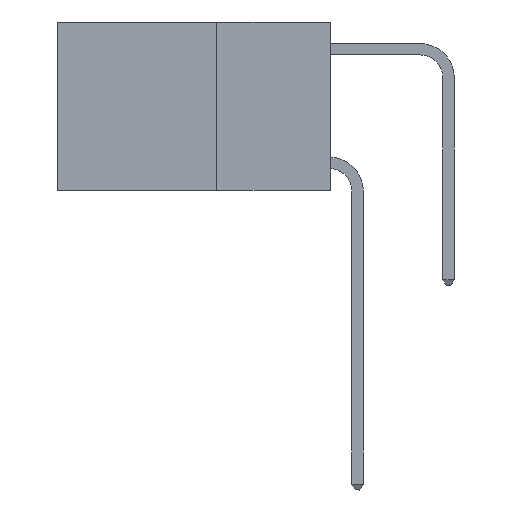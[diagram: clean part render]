
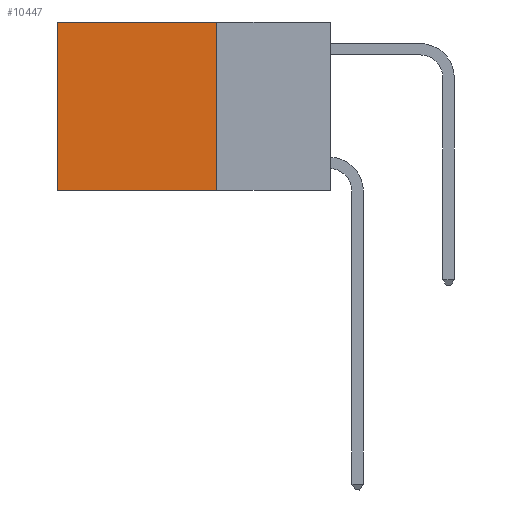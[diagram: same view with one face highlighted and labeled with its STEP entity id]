
A CAD part, left-side view. The second image highlights one B-rep face of the part: STEP entity #10447.
In plain terms, the highlighted planar face has unit normal (-1, 0, 0).
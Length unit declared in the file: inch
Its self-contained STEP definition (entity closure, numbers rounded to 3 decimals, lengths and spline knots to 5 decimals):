
#599 = DIRECTION ( 'NONE',  ( 0., 0., -1. ) ) ;
#1930 = VECTOR ( 'NONE', #29055, 39.37008 ) ;
#3111 = AXIS2_PLACEMENT_3D ( 'NONE', #27668, #14146, #599 ) ;
#3368 = VECTOR ( 'NONE', #26157, 39.37008 ) ;
#3577 = VERTEX_POINT ( 'NONE', #8261 ) ;
#4535 = CARTESIAN_POINT ( 'NONE',  ( 0.2625, 0.6, 0. ) ) ;
#6037 = LINE ( 'NONE', #8114, #6746 ) ;
#6746 = VECTOR ( 'NONE', #10373, 39.37008 ) ;
#7143 = EDGE_CURVE ( 'NONE', #3577, #18643, #6037, .T. ) ;
#8114 = CARTESIAN_POINT ( 'NONE',  ( 0.2625, 0.25, -0.37 ) ) ;
#8261 = CARTESIAN_POINT ( 'NONE',  ( 0.2625, 0.25, -0.37 ) ) ;
#8623 = LINE ( 'NONE', #24556, #1930 ) ;
#9758 = VERTEX_POINT ( 'NONE', #14080 ) ;
#10373 = DIRECTION ( 'NONE',  ( 0., 1., 0. ) ) ;
#10447 = ADVANCED_FACE ( 'NONE', ( #15789 ), #25421, .F. ) ;
#11346 = ORIENTED_EDGE ( 'NONE', *, *, #27672, .F. ) ;
#11373 = EDGE_CURVE ( 'NONE', #9758, #15283, #27414, .T. ) ;
#12584 = CARTESIAN_POINT ( 'NONE',  ( 0.2625, 0.25, 0. ) ) ;
#13451 = EDGE_CURVE ( 'NONE', #15283, #18643, #8623, .T. ) ;
#14080 = CARTESIAN_POINT ( 'NONE',  ( 0.2625, 0.25, 0. ) ) ;
#14122 = VECTOR ( 'NONE', #17530, 39.37008 ) ;
#14146 = DIRECTION ( 'NONE',  ( 1., 0., 0. ) ) ;
#15283 = VERTEX_POINT ( 'NONE', #4535 ) ;
#15789 = FACE_OUTER_BOUND ( 'NONE', #20632, .T. ) ;
#17530 = DIRECTION ( 'NONE',  ( 0., 0., -1. ) ) ;
#18643 = VERTEX_POINT ( 'NONE', #26616 ) ;
#19756 = ORIENTED_EDGE ( 'NONE', *, *, #11373, .T. ) ;
#20632 = EDGE_LOOP ( 'NONE', ( #28697, #26575, #11346, #19756 ) ) ;
#24556 = CARTESIAN_POINT ( 'NONE',  ( 0.2625, 0.6, 0. ) ) ;
#25421 = PLANE ( 'NONE',  #3111 ) ;
#26142 = LINE ( 'NONE', #26517, #14122 ) ;
#26157 = DIRECTION ( 'NONE',  ( 0., 1., 0. ) ) ;
#26517 = CARTESIAN_POINT ( 'NONE',  ( 0.2625, 0.25, 0. ) ) ;
#26575 = ORIENTED_EDGE ( 'NONE', *, *, #7143, .F. ) ;
#26616 = CARTESIAN_POINT ( 'NONE',  ( 0.2625, 0.6, -0.37 ) ) ;
#27414 = LINE ( 'NONE', #12584, #3368 ) ;
#27668 = CARTESIAN_POINT ( 'NONE',  ( 0.2625, 0.25, 0. ) ) ;
#27672 = EDGE_CURVE ( 'NONE', #9758, #3577, #26142, .T. ) ;
#28697 = ORIENTED_EDGE ( 'NONE', *, *, #13451, .T. ) ;
#29055 = DIRECTION ( 'NONE',  ( 0., 0., -1. ) ) ;
